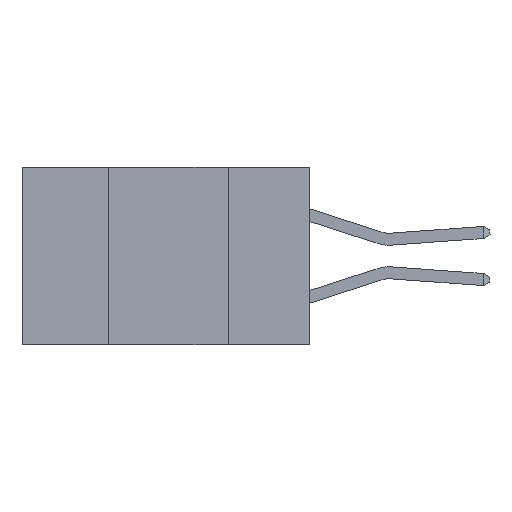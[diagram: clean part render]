
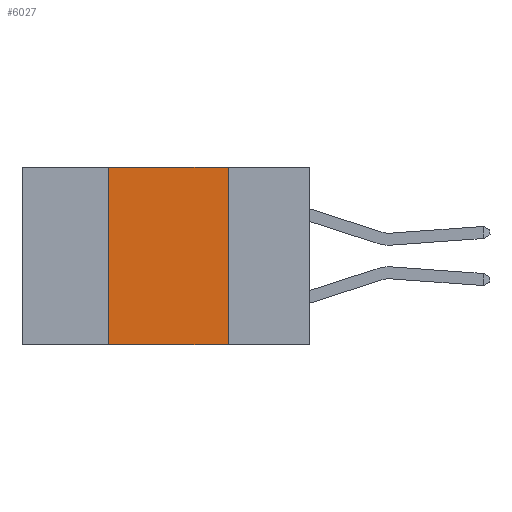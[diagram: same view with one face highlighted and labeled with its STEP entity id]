
A CAD part, left-side view. The second image highlights one B-rep face of the part: STEP entity #6027.
In plain terms, the highlighted planar face has unit normal (-1, 0, 0).
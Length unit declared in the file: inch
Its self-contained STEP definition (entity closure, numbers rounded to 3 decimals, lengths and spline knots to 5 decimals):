
#196 = DIRECTION ( 'NONE',  ( 0., 0., 1. ) ) ;
#204 = LINE ( 'NONE', #5372, #1595 ) ;
#317 = DIRECTION ( 'NONE',  ( 0., 0., -1. ) ) ;
#683 = EDGE_CURVE ( 'NONE', #5304, #4711, #9959, .T. ) ;
#1143 = DIRECTION ( 'NONE',  ( 0., 0., -1. ) ) ;
#1275 = EDGE_LOOP ( 'NONE', ( #2641, #3747, #3046, #9926 ) ) ;
#1439 = DIRECTION ( 'NONE',  ( 0., -1., 0. ) ) ;
#1595 = VECTOR ( 'NONE', #1439, 39.37008 ) ;
#2276 = CARTESIAN_POINT ( 'NONE',  ( 0., 0.17, 0. ) ) ;
#2463 = VECTOR ( 'NONE', #1143, 39.37008 ) ;
#2641 = ORIENTED_EDGE ( 'NONE', *, *, #683, .F. ) ;
#2689 = VECTOR ( 'NONE', #196, 39.37008 ) ;
#3046 = ORIENTED_EDGE ( 'NONE', *, *, #5413, .F. ) ;
#3562 = DIRECTION ( 'NONE',  ( 0., -1., 0. ) ) ;
#3619 = CARTESIAN_POINT ( 'NONE',  ( 0., 0.42, 0. ) ) ;
#3709 = VECTOR ( 'NONE', #3562, 39.37008 ) ;
#3747 = ORIENTED_EDGE ( 'NONE', *, *, #8122, .F. ) ;
#4016 = LINE ( 'NONE', #9407, #3709 ) ;
#4105 = VERTEX_POINT ( 'NONE', #12179 ) ;
#4240 = PLANE ( 'NONE',  #11129 ) ;
#4617 = VERTEX_POINT ( 'NONE', #5380 ) ;
#4711 = VERTEX_POINT ( 'NONE', #8050 ) ;
#5304 = VERTEX_POINT ( 'NONE', #9620 ) ;
#5372 = CARTESIAN_POINT ( 'NONE',  ( 0., 0.6, -0.37 ) ) ;
#5380 = CARTESIAN_POINT ( 'NONE',  ( 0., 0.42, -0.37 ) ) ;
#5413 = EDGE_CURVE ( 'NONE', #4617, #4105, #11097, .T. ) ;
#6027 = ADVANCED_FACE ( 'NONE', ( #8077 ), #4240, .F. ) ;
#6130 = EDGE_CURVE ( 'NONE', #4617, #4711, #204, .T. ) ;
#6213 = DIRECTION ( 'NONE',  ( 1., 0., 0. ) ) ;
#8050 = CARTESIAN_POINT ( 'NONE',  ( 0., 0.17, -0.37 ) ) ;
#8077 = FACE_OUTER_BOUND ( 'NONE', #1275, .T. ) ;
#8122 = EDGE_CURVE ( 'NONE', #4105, #5304, #4016, .T. ) ;
#9407 = CARTESIAN_POINT ( 'NONE',  ( 0., 0.6, 0. ) ) ;
#9620 = CARTESIAN_POINT ( 'NONE',  ( 0., 0.17, 0. ) ) ;
#9926 = ORIENTED_EDGE ( 'NONE', *, *, #6130, .T. ) ;
#9959 = LINE ( 'NONE', #2276, #2463 ) ;
#11097 = LINE ( 'NONE', #3619, #2689 ) ;
#11129 = AXIS2_PLACEMENT_3D ( 'NONE', #12040, #6213, #317 ) ;
#12040 = CARTESIAN_POINT ( 'NONE',  ( 0., 0.6, 0. ) ) ;
#12179 = CARTESIAN_POINT ( 'NONE',  ( 0., 0.42, 0. ) ) ;
